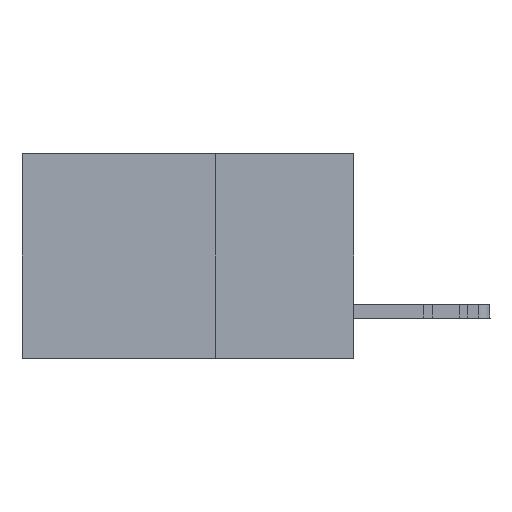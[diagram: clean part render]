
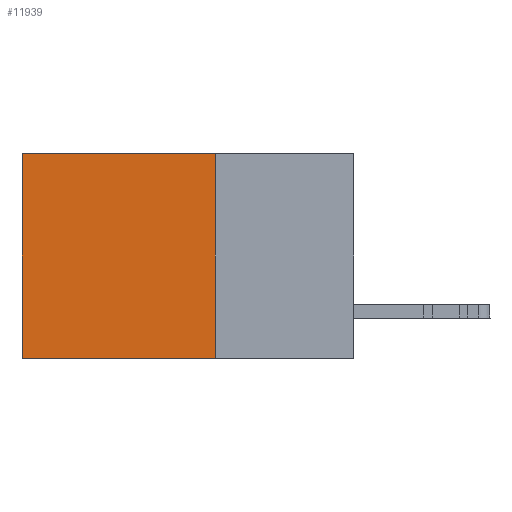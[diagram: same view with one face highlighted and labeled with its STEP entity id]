
A CAD part, left-side view. The second image highlights one B-rep face of the part: STEP entity #11939.
In plain terms, the highlighted planar face has unit normal (-1, 0, 0).
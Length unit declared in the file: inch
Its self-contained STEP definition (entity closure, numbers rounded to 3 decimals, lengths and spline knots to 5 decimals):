
#642 = DIRECTION ( 'NONE',  ( 0., 1., 0. ) ) ;
#1318 = EDGE_CURVE ( 'NONE', #8903, #2177, #16330, .T. ) ;
#1775 = CARTESIAN_POINT ( 'NONE',  ( 0.2875, 0.25, 0. ) ) ;
#2177 = VERTEX_POINT ( 'NONE', #42634 ) ;
#3222 = ORIENTED_EDGE ( 'NONE', *, *, #1318, .T. ) ;
#3458 = LINE ( 'NONE', #4223, #8486 ) ;
#4073 = AXIS2_PLACEMENT_3D ( 'NONE', #45673, #20580, #46347 ) ;
#4223 = CARTESIAN_POINT ( 'NONE',  ( 0.2875, 0.25, 0. ) ) ;
#5566 = EDGE_LOOP ( 'NONE', ( #27515, #45793, #22235, #3222 ) ) ;
#6146 = FACE_OUTER_BOUND ( 'NONE', #5566, .T. ) ;
#7869 = VECTOR ( 'NONE', #642, 39.37008 ) ;
#8486 = VECTOR ( 'NONE', #30301, 39.37008 ) ;
#8903 = VERTEX_POINT ( 'NONE', #47538 ) ;
#11939 = ADVANCED_FACE ( 'NONE', ( #6146 ), #46004, .F. ) ;
#13425 = DIRECTION ( 'NONE',  ( 0., 1., 0. ) ) ;
#14930 = LINE ( 'NONE', #19087, #7869 ) ;
#16330 = LINE ( 'NONE', #1775, #25099 ) ;
#19087 = CARTESIAN_POINT ( 'NONE',  ( 0.2875, 0.25, -0.37 ) ) ;
#20580 = DIRECTION ( 'NONE',  ( 1., 0., 0. ) ) ;
#21233 = VERTEX_POINT ( 'NONE', #32108 ) ;
#22235 = ORIENTED_EDGE ( 'NONE', *, *, #42318, .F. ) ;
#23705 = VECTOR ( 'NONE', #26350, 39.37008 ) ;
#25099 = VECTOR ( 'NONE', #13425, 39.37008 ) ;
#26350 = DIRECTION ( 'NONE',  ( 0., 0., -1. ) ) ;
#27386 = EDGE_CURVE ( 'NONE', #2177, #44476, #33621, .T. ) ;
#27515 = ORIENTED_EDGE ( 'NONE', *, *, #27386, .T. ) ;
#30301 = DIRECTION ( 'NONE',  ( 0., 0., -1. ) ) ;
#32108 = CARTESIAN_POINT ( 'NONE',  ( 0.2875, 0.25, -0.37 ) ) ;
#33621 = LINE ( 'NONE', #36861, #23705 ) ;
#36861 = CARTESIAN_POINT ( 'NONE',  ( 0.2875, 0.6, 0. ) ) ;
#42261 = EDGE_CURVE ( 'NONE', #21233, #44476, #14930, .T. ) ;
#42318 = EDGE_CURVE ( 'NONE', #8903, #21233, #3458, .T. ) ;
#42634 = CARTESIAN_POINT ( 'NONE',  ( 0.2875, 0.6, 0. ) ) ;
#44214 = CARTESIAN_POINT ( 'NONE',  ( 0.2875, 0.6, -0.37 ) ) ;
#44476 = VERTEX_POINT ( 'NONE', #44214 ) ;
#45673 = CARTESIAN_POINT ( 'NONE',  ( 0.2875, 0.25, 0. ) ) ;
#45793 = ORIENTED_EDGE ( 'NONE', *, *, #42261, .F. ) ;
#46004 = PLANE ( 'NONE',  #4073 ) ;
#46347 = DIRECTION ( 'NONE',  ( 0., 0., -1. ) ) ;
#47538 = CARTESIAN_POINT ( 'NONE',  ( 0.2875, 0.25, 0. ) ) ;
